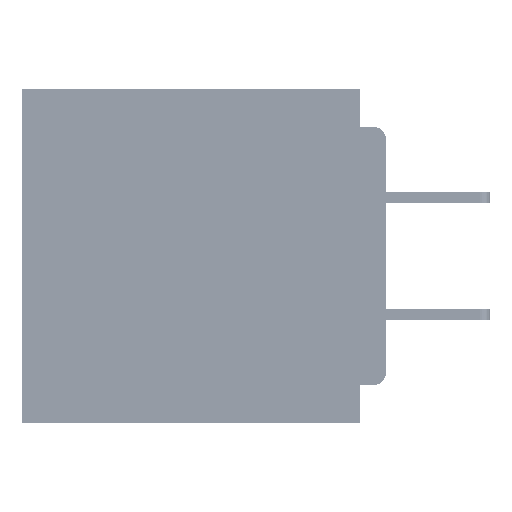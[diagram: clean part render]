
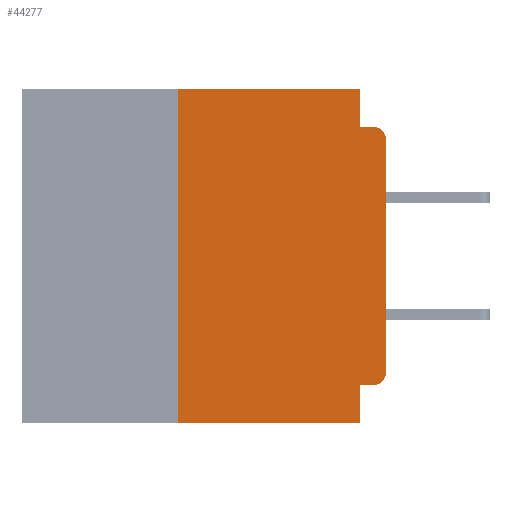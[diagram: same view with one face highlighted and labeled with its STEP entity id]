
A CAD part, left-side view. The second image highlights one B-rep face of the part: STEP entity #44277.
In plain terms, the highlighted planar face has unit normal (-1, 0, 0).
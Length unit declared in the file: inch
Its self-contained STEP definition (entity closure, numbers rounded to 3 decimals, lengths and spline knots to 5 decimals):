
#729 = DIRECTION ( 'NONE',  ( -1., 0., 0. ) ) ;
#1041 = VERTEX_POINT ( 'NONE', #6820 ) ;
#2442 = CARTESIAN_POINT ( 'NONE',  ( 0., 0.25, -0.4 ) ) ;
#2912 = EDGE_CURVE ( 'NONE', #34362, #51859, #64130, .T. ) ;
#3941 = DIRECTION ( 'NONE',  ( 1., 0., 0. ) ) ;
#6039 = CARTESIAN_POINT ( 'NONE',  ( 0., 0., -0.34 ) ) ;
#6820 = CARTESIAN_POINT ( 'NONE',  ( 0., 0.031, -0.045 ) ) ;
#7752 = VERTEX_POINT ( 'NONE', #48985 ) ;
#8124 = CARTESIAN_POINT ( 'NONE',  ( 0., 0.031, -0.4 ) ) ;
#9118 = VERTEX_POINT ( 'NONE', #43826 ) ;
#10877 = CIRCLE ( 'NONE', #54945, 0.015 ) ;
#11302 = EDGE_CURVE ( 'NONE', #7752, #34782, #57004, .T. ) ;
#11977 = AXIS2_PLACEMENT_3D ( 'NONE', #35583, #3941, #40884 ) ;
#14265 = ORIENTED_EDGE ( 'NONE', *, *, #28353, .F. ) ;
#14990 = CARTESIAN_POINT ( 'NONE',  ( 0., 0., -0.355 ) ) ;
#15184 = LINE ( 'NONE', #14990, #67745 ) ;
#15743 = EDGE_CURVE ( 'NONE', #7752, #52467, #19300, .T. ) ;
#16253 = CARTESIAN_POINT ( 'NONE',  ( 0., 0.031, -0.4 ) ) ;
#16450 = CARTESIAN_POINT ( 'NONE',  ( 0., 0., -0.045 ) ) ;
#17522 = ORIENTED_EDGE ( 'NONE', *, *, #35161, .T. ) ;
#18727 = CARTESIAN_POINT ( 'NONE',  ( 0., 0.437, 0. ) ) ;
#19300 = LINE ( 'NONE', #2442, #61241 ) ;
#21082 = CARTESIAN_POINT ( 'NONE',  ( 0., 0., -0.06 ) ) ;
#21779 = FACE_OUTER_BOUND ( 'NONE', #42240, .T. ) ;
#22830 = DIRECTION ( 'NONE',  ( 0., 0., -1. ) ) ;
#22900 = DIRECTION ( 'NONE',  ( -1., 0., 0. ) ) ;
#22921 = DIRECTION ( 'NONE',  ( 0., -1., 0. ) ) ;
#23005 = CARTESIAN_POINT ( 'NONE',  ( 0., 0.015, -0.06 ) ) ;
#23263 = CARTESIAN_POINT ( 'NONE',  ( 0., 0.015, -0.045 ) ) ;
#24873 = EDGE_CURVE ( 'NONE', #9118, #1041, #62449, .T. ) ;
#25029 = ORIENTED_EDGE ( 'NONE', *, *, #36486, .F. ) ;
#25301 = VECTOR ( 'NONE', #47575, 39.37008 ) ;
#27306 = CARTESIAN_POINT ( 'NONE',  ( 0., 0.031, -0.355 ) ) ;
#28314 = DIRECTION ( 'NONE',  ( 0., 0., -1. ) ) ;
#28353 = EDGE_CURVE ( 'NONE', #39749, #32695, #15184, .T. ) ;
#28758 = VECTOR ( 'NONE', #53055, 39.37008 ) ;
#30387 = LINE ( 'NONE', #16253, #28758 ) ;
#30741 = VECTOR ( 'NONE', #22921, 39.37008 ) ;
#32141 = DIRECTION ( 'NONE',  ( 0., -1., 0. ) ) ;
#32305 = CARTESIAN_POINT ( 'NONE',  ( 0., 0.015, -0.34 ) ) ;
#32637 = ORIENTED_EDGE ( 'NONE', *, *, #62075, .T. ) ;
#32695 = VERTEX_POINT ( 'NONE', #27306 ) ;
#34067 = DIRECTION ( 'NONE',  ( 0., 0., 1. ) ) ;
#34362 = VERTEX_POINT ( 'NONE', #21082 ) ;
#34782 = VERTEX_POINT ( 'NONE', #8124 ) ;
#35161 = EDGE_CURVE ( 'NONE', #39749, #36500, #10877, .T. ) ;
#35583 = CARTESIAN_POINT ( 'NONE',  ( 0., 0.437, 0. ) ) ;
#36198 = DIRECTION ( 'NONE',  ( 0., 1., 0. ) ) ;
#36486 = EDGE_CURVE ( 'NONE', #1041, #51859, #40788, .T. ) ;
#36500 = VERTEX_POINT ( 'NONE', #6039 ) ;
#37602 = DIRECTION ( 'NONE',  ( 0., 0., -1. ) ) ;
#39749 = VERTEX_POINT ( 'NONE', #40540 ) ;
#39963 = LINE ( 'NONE', #18727, #67728 ) ;
#40540 = CARTESIAN_POINT ( 'NONE',  ( 0., 0.015, -0.355 ) ) ;
#40788 = LINE ( 'NONE', #16450, #66936 ) ;
#40884 = DIRECTION ( 'NONE',  ( 0., 0., -1. ) ) ;
#42240 = EDGE_LOOP ( 'NONE', ( #32637, #61219, #25029, #53095, #61201, #53894, #49781, #48804, #14265, #17522 ) ) ;
#43826 = CARTESIAN_POINT ( 'NONE',  ( 0., 0.031, 0. ) ) ;
#44277 = ADVANCED_FACE ( 'NONE', ( #21779 ), #51182, .F. ) ;
#46911 = VECTOR ( 'NONE', #28314, 39.37008 ) ;
#47575 = DIRECTION ( 'NONE',  ( 0., 0., 1. ) ) ;
#48804 = ORIENTED_EDGE ( 'NONE', *, *, #52279, .F. ) ;
#48985 = CARTESIAN_POINT ( 'NONE',  ( 0., 0.25, -0.4 ) ) ;
#49437 = CARTESIAN_POINT ( 'NONE',  ( 0., 0.031, 0. ) ) ;
#49781 = ORIENTED_EDGE ( 'NONE', *, *, #11302, .T. ) ;
#50256 = DIRECTION ( 'NONE',  ( 0., -1., 0. ) ) ;
#51182 = PLANE ( 'NONE',  #11977 ) ;
#51362 = AXIS2_PLACEMENT_3D ( 'NONE', #23005, #22900, #22830 ) ;
#51859 = VERTEX_POINT ( 'NONE', #23263 ) ;
#52279 = EDGE_CURVE ( 'NONE', #32695, #34782, #30387, .T. ) ;
#52467 = VERTEX_POINT ( 'NONE', #54871 ) ;
#52614 = CARTESIAN_POINT ( 'NONE',  ( 0., 0., 0. ) ) ;
#53055 = DIRECTION ( 'NONE',  ( 0., 0., -1. ) ) ;
#53095 = ORIENTED_EDGE ( 'NONE', *, *, #24873, .F. ) ;
#53236 = LINE ( 'NONE', #52614, #25301 ) ;
#53894 = ORIENTED_EDGE ( 'NONE', *, *, #15743, .F. ) ;
#54402 = CARTESIAN_POINT ( 'NONE',  ( 0., 0.437, -0.4 ) ) ;
#54871 = CARTESIAN_POINT ( 'NONE',  ( 0., 0.25, 0. ) ) ;
#54945 = AXIS2_PLACEMENT_3D ( 'NONE', #32305, #729, #37602 ) ;
#57004 = LINE ( 'NONE', #54402, #30741 ) ;
#61201 = ORIENTED_EDGE ( 'NONE', *, *, #67645, .F. ) ;
#61219 = ORIENTED_EDGE ( 'NONE', *, *, #2912, .T. ) ;
#61241 = VECTOR ( 'NONE', #34067, 39.37008 ) ;
#62075 = EDGE_CURVE ( 'NONE', #36500, #34362, #53236, .T. ) ;
#62449 = LINE ( 'NONE', #49437, #46911 ) ;
#64130 = CIRCLE ( 'NONE', #51362, 0.015 ) ;
#66936 = VECTOR ( 'NONE', #32141, 39.37008 ) ;
#67645 = EDGE_CURVE ( 'NONE', #52467, #9118, #39963, .T. ) ;
#67728 = VECTOR ( 'NONE', #50256, 39.37008 ) ;
#67745 = VECTOR ( 'NONE', #36198, 39.37008 ) ;
